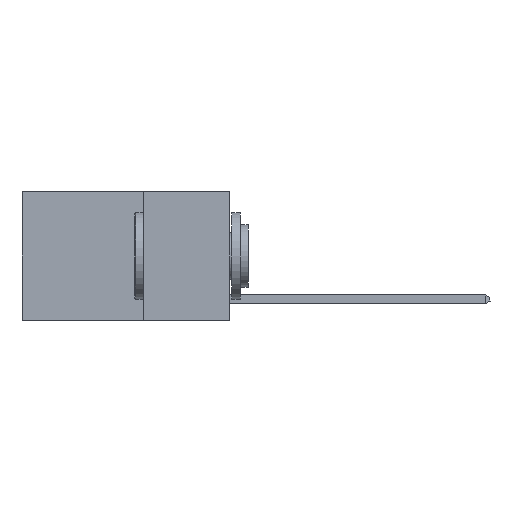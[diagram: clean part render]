
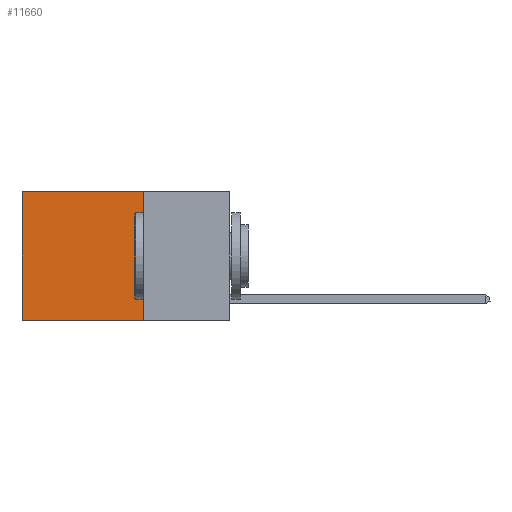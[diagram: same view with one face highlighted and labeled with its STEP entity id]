
A CAD part, left-side view. The second image highlights one B-rep face of the part: STEP entity #11660.
In plain terms, the highlighted planar face has unit normal (-1, 0, 0).
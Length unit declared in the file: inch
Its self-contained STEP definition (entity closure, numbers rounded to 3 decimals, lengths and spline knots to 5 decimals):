
#2 = CARTESIAN_POINT ( 'NONE',  ( 0.2625, 0.25, 0. ) ) ;
#3772 = VECTOR ( 'NONE', #8384, 39.37008 ) ;
#4582 = CARTESIAN_POINT ( 'NONE',  ( 0.2625, 0.6, 0. ) ) ;
#5397 = PLANE ( 'NONE',  #10110 ) ;
#5495 = LINE ( 'NONE', #2, #10395 ) ;
#5499 = VECTOR ( 'NONE', #8214, 39.37008 ) ;
#6451 = CARTESIAN_POINT ( 'NONE',  ( 0.2625, 0.25, 0. ) ) ;
#6656 = LINE ( 'NONE', #19236, #5499 ) ;
#6851 = FACE_OUTER_BOUND ( 'NONE', #13894, .T. ) ;
#7031 = DIRECTION ( 'NONE',  ( 0., 1., 0. ) ) ;
#7231 = DIRECTION ( 'NONE',  ( 0., 0., -1. ) ) ;
#7493 = EDGE_CURVE ( 'NONE', #11289, #9357, #23427, .T. ) ;
#8214 = DIRECTION ( 'NONE',  ( 0., 0., -1. ) ) ;
#8384 = DIRECTION ( 'NONE',  ( 0., 1., 0. ) ) ;
#9232 = LINE ( 'NONE', #6451, #3772 ) ;
#9357 = VERTEX_POINT ( 'NONE', #16266 ) ;
#10110 = AXIS2_PLACEMENT_3D ( 'NONE', #16403, #18272, #7231 ) ;
#10395 = VECTOR ( 'NONE', #11065, 39.37008 ) ;
#11065 = DIRECTION ( 'NONE',  ( 0., 0., -1. ) ) ;
#11289 = VERTEX_POINT ( 'NONE', #18917 ) ;
#11660 = ADVANCED_FACE ( 'NONE', ( #6851 ), #5397, .F. ) ;
#11756 = VERTEX_POINT ( 'NONE', #16646 ) ;
#12477 = ORIENTED_EDGE ( 'NONE', *, *, #17742, .T. ) ;
#13125 = VERTEX_POINT ( 'NONE', #4582 ) ;
#13894 = EDGE_LOOP ( 'NONE', ( #12477, #16683, #22283, #19711 ) ) ;
#16266 = CARTESIAN_POINT ( 'NONE',  ( 0.2625, 0.6, -0.37 ) ) ;
#16403 = CARTESIAN_POINT ( 'NONE',  ( 0.2625, 0.25, 0. ) ) ;
#16646 = CARTESIAN_POINT ( 'NONE',  ( 0.2625, 0.25, 0. ) ) ;
#16683 = ORIENTED_EDGE ( 'NONE', *, *, #7493, .F. ) ;
#17742 = EDGE_CURVE ( 'NONE', #13125, #9357, #6656, .T. ) ;
#17803 = EDGE_CURVE ( 'NONE', #11756, #13125, #9232, .T. ) ;
#18272 = DIRECTION ( 'NONE',  ( 1., 0., 0. ) ) ;
#18917 = CARTESIAN_POINT ( 'NONE',  ( 0.2625, 0.25, -0.37 ) ) ;
#19125 = VECTOR ( 'NONE', #7031, 39.37008 ) ;
#19236 = CARTESIAN_POINT ( 'NONE',  ( 0.2625, 0.6, 0. ) ) ;
#19711 = ORIENTED_EDGE ( 'NONE', *, *, #17803, .T. ) ;
#19810 = EDGE_CURVE ( 'NONE', #11756, #11289, #5495, .T. ) ;
#19880 = CARTESIAN_POINT ( 'NONE',  ( 0.2625, 0.25, -0.37 ) ) ;
#22283 = ORIENTED_EDGE ( 'NONE', *, *, #19810, .F. ) ;
#23427 = LINE ( 'NONE', #19880, #19125 ) ;
